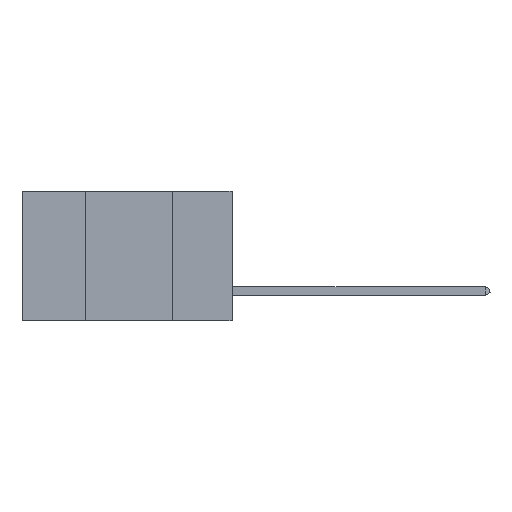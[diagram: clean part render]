
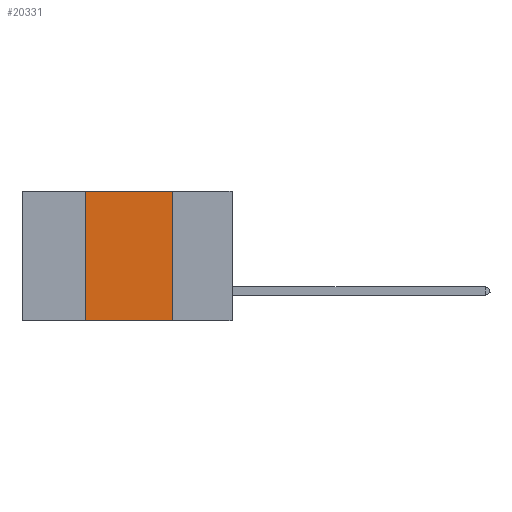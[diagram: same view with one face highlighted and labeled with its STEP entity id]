
A CAD part, left-side view. The second image highlights one B-rep face of the part: STEP entity #20331.
In plain terms, the highlighted planar face has unit normal (-1, 0, 0).
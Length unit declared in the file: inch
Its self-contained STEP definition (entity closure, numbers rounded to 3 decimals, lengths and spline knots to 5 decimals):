
#1944 = CARTESIAN_POINT ( 'NONE',  ( 0., 0.17, 0. ) ) ;
#2101 = VECTOR ( 'NONE', #9950, 39.37008 ) ;
#3249 = CARTESIAN_POINT ( 'NONE',  ( 0., 0.42, -0.37 ) ) ;
#3765 = CARTESIAN_POINT ( 'NONE',  ( 0., 0.6, 0. ) ) ;
#5817 = VERTEX_POINT ( 'NONE', #11948 ) ;
#6153 = VERTEX_POINT ( 'NONE', #3249 ) ;
#6507 = EDGE_CURVE ( 'NONE', #6153, #13176, #26532, .T. ) ;
#7075 = VECTOR ( 'NONE', #16993, 39.37008 ) ;
#7263 = CARTESIAN_POINT ( 'NONE',  ( 0., 0.6, 0. ) ) ;
#8467 = DIRECTION ( 'NONE',  ( 0., 0., -1. ) ) ;
#8781 = VERTEX_POINT ( 'NONE', #8927 ) ;
#8927 = CARTESIAN_POINT ( 'NONE',  ( 0., 0.17, 0. ) ) ;
#9950 = DIRECTION ( 'NONE',  ( 0., -1., 0. ) ) ;
#10268 = LINE ( 'NONE', #7263, #7075 ) ;
#11948 = CARTESIAN_POINT ( 'NONE',  ( 0., 0.17, -0.37 ) ) ;
#13176 = VERTEX_POINT ( 'NONE', #20090 ) ;
#13895 = DIRECTION ( 'NONE',  ( 1., 0., 0. ) ) ;
#13916 = VECTOR ( 'NONE', #29851, 39.37008 ) ;
#16756 = ORIENTED_EDGE ( 'NONE', *, *, #19916, .F. ) ;
#16929 = EDGE_CURVE ( 'NONE', #6153, #5817, #28248, .T. ) ;
#16993 = DIRECTION ( 'NONE',  ( 0., -1., 0. ) ) ;
#17271 = DIRECTION ( 'NONE',  ( 0., 0., 1. ) ) ;
#19916 = EDGE_CURVE ( 'NONE', #13176, #8781, #10268, .T. ) ;
#20090 = CARTESIAN_POINT ( 'NONE',  ( 0., 0.42, 0. ) ) ;
#20331 = ADVANCED_FACE ( 'NONE', ( #29173 ), #28664, .F. ) ;
#22409 = CARTESIAN_POINT ( 'NONE',  ( 0., 0.6, -0.37 ) ) ;
#22957 = VECTOR ( 'NONE', #17271, 39.37008 ) ;
#24566 = LINE ( 'NONE', #1944, #13916 ) ;
#26532 = LINE ( 'NONE', #26660, #22957 ) ;
#26660 = CARTESIAN_POINT ( 'NONE',  ( 0., 0.42, 0. ) ) ;
#28248 = LINE ( 'NONE', #22409, #2101 ) ;
#28283 = ORIENTED_EDGE ( 'NONE', *, *, #16929, .T. ) ;
#28664 = PLANE ( 'NONE',  #29899 ) ;
#29173 = FACE_OUTER_BOUND ( 'NONE', #30417, .T. ) ;
#29249 = ORIENTED_EDGE ( 'NONE', *, *, #29436, .F. ) ;
#29436 = EDGE_CURVE ( 'NONE', #8781, #5817, #24566, .T. ) ;
#29851 = DIRECTION ( 'NONE',  ( 0., 0., -1. ) ) ;
#29855 = ORIENTED_EDGE ( 'NONE', *, *, #6507, .F. ) ;
#29899 = AXIS2_PLACEMENT_3D ( 'NONE', #3765, #13895, #8467 ) ;
#30417 = EDGE_LOOP ( 'NONE', ( #29249, #16756, #29855, #28283 ) ) ;
